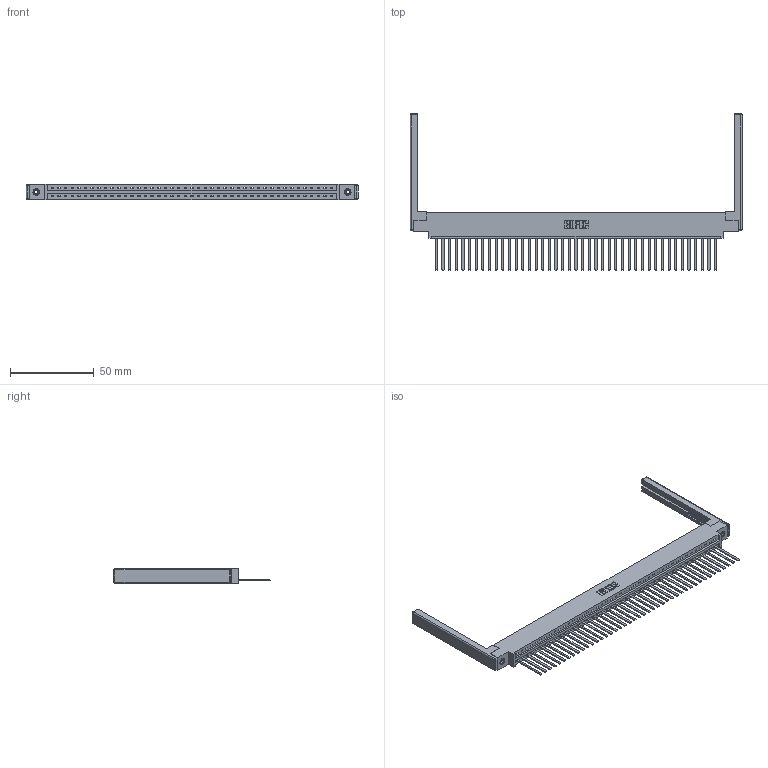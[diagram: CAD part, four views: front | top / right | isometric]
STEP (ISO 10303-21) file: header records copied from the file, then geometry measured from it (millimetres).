
FILE_DESCRIPTION (( 'STEP AP203' ), '1' );
FILE_NAME ('337-043-544-668.STEP', '2019-10-02T00:06:45', ( '' ), ( '' ), 'SwSTEP 2.0', 'SolidWorks 2016', '' );
FILE_SCHEMA (( 'CONFIG_CONTROL_DESIGN' ));
Length unit declared in the file: inch
Products named in the file (5): 337-043-544-668; 345-292-001_345-293-144; 337 Part_0.170 Offset - 0.156 Dia-TI; 345-250-001_345-250-001-102; 307-220-068
Assembly tree (48 placements, depth 2):
  337-043-544-668
    337 Part_0.170 Offset - 0.156 Dia-TI
    345-292-001_345-293-144  x43
    345-250-001_345-250-001-102  x2
    307-220-068  x2
Bounding box: 197.82 x 93.35 x 9.4 mm (x, y, z)
Volume: 25343.8 mm3; surface area: 27484.2 mm2
Topology: 48 solids, 48 shells, 2680 faces, 8023 edges, 5270 vertices
Faces by surface type: plane 1968, cylinder 688, cone 12, sphere 8, torus 4
Entity records: 34542 total; most frequent: CARTESIAN_POINT 5972, ORIENTED_EDGE 5940, DIRECTION 5094, EDGE_CURVE 2970, VECTOR 2796, LINE 2796, VERTEX_POINT 1970, AXIS2_PLACEMENT_3D 1149
